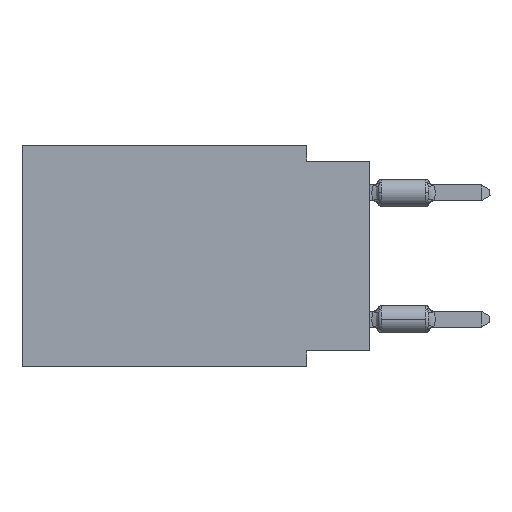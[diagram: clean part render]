
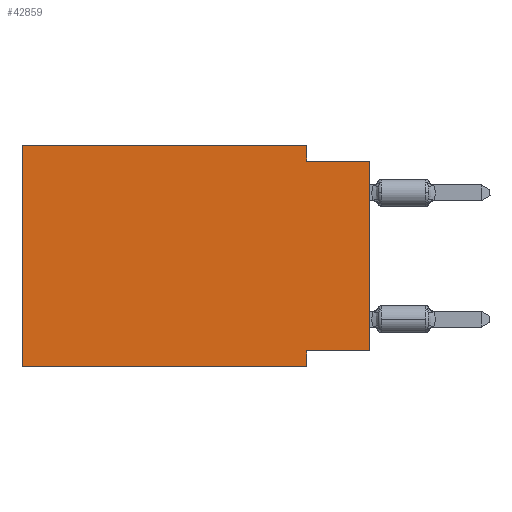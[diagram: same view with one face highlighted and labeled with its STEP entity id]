
A CAD part, left-side view. The second image highlights one B-rep face of the part: STEP entity #42859.
In plain terms, the highlighted planar face has unit normal (-1, 0, 0).
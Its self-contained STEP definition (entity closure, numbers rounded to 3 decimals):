
#439 = VERTEX_POINT ( 'NONE', #24059 ) ;
#2502 = EDGE_CURVE ( 'NONE', #50353, #28682, #31240, .T. ) ;
#2785 = CARTESIAN_POINT ( 'NONE',  ( 0., 0., 0. ) ) ;
#2796 = CARTESIAN_POINT ( 'NONE',  ( 0., 13.97, 0. ) ) ;
#3063 = AXIS2_PLACEMENT_3D ( 'NONE', #2796, #46079, #18125 ) ;
#3185 = CARTESIAN_POINT ( 'NONE',  ( 0., 0., -8.255 ) ) ;
#4720 = EDGE_CURVE ( 'NONE', #48730, #28686, #17129, .T. ) ;
#4770 = CARTESIAN_POINT ( 'NONE',  ( 0., 2.54, -0.635 ) ) ;
#7696 = EDGE_CURVE ( 'NONE', #50228, #50353, #31667, .T. ) ;
#11003 = LINE ( 'NONE', #39218, #25266 ) ;
#14453 = CARTESIAN_POINT ( 'NONE',  ( 0., 13.97, 0. ) ) ;
#14509 = VECTOR ( 'NONE', #24447, 1000. ) ;
#15107 = LINE ( 'NONE', #31175, #27765 ) ;
#17129 = LINE ( 'NONE', #45602, #43668 ) ;
#18125 = DIRECTION ( 'NONE',  ( 0., 0., -1. ) ) ;
#22542 = ORIENTED_EDGE ( 'NONE', *, *, #4720, .F. ) ;
#24059 = CARTESIAN_POINT ( 'NONE',  ( 0., 0., -0.635 ) ) ;
#24447 = DIRECTION ( 'NONE',  ( 0., -1., 0. ) ) ;
#24557 = ORIENTED_EDGE ( 'NONE', *, *, #34786, .F. ) ;
#25266 = VECTOR ( 'NONE', #31302, 1000. ) ;
#25307 = CARTESIAN_POINT ( 'NONE',  ( 0., 13.97, -8.89 ) ) ;
#27765 = VECTOR ( 'NONE', #47256, 1000. ) ;
#28682 = VERTEX_POINT ( 'NONE', #49790 ) ;
#28686 = VERTEX_POINT ( 'NONE', #14453 ) ;
#29984 = FACE_OUTER_BOUND ( 'NONE', #46580, .T. ) ;
#30478 = DIRECTION ( 'NONE',  ( 0., 0., 1. ) ) ;
#31080 = EDGE_CURVE ( 'NONE', #48730, #28682, #40788, .T. ) ;
#31090 = ORIENTED_EDGE ( 'NONE', *, *, #33074, .F. ) ;
#31175 = CARTESIAN_POINT ( 'NONE',  ( 0., 2.54, 0. ) ) ;
#31240 = LINE ( 'NONE', #50745, #32575 ) ;
#31302 = DIRECTION ( 'NONE',  ( 0., -1., 0. ) ) ;
#31667 = LINE ( 'NONE', #3185, #40478 ) ;
#32575 = VECTOR ( 'NONE', #46552, 1000. ) ;
#33074 = EDGE_CURVE ( 'NONE', #28686, #51881, #40324, .T. ) ;
#33161 = VECTOR ( 'NONE', #47181, 1000. ) ;
#33210 = DIRECTION ( 'NONE',  ( 0., 0., 1. ) ) ;
#34425 = EDGE_CURVE ( 'NONE', #51881, #49497, #15107, .T. ) ;
#34786 = EDGE_CURVE ( 'NONE', #49497, #439, #11003, .T. ) ;
#38143 = LINE ( 'NONE', #2785, #42361 ) ;
#38491 = ORIENTED_EDGE ( 'NONE', *, *, #7696, .F. ) ;
#39218 = CARTESIAN_POINT ( 'NONE',  ( 0., 0., -0.635 ) ) ;
#39727 = CARTESIAN_POINT ( 'NONE',  ( 0., 2.54, -8.255 ) ) ;
#40324 = LINE ( 'NONE', #51388, #33161 ) ;
#40423 = EDGE_CURVE ( 'NONE', #50228, #439, #38143, .T. ) ;
#40478 = VECTOR ( 'NONE', #42759, 1000. ) ;
#40562 = ORIENTED_EDGE ( 'NONE', *, *, #34425, .F. ) ;
#40788 = LINE ( 'NONE', #44490, #14509 ) ;
#42361 = VECTOR ( 'NONE', #30478, 1000. ) ;
#42759 = DIRECTION ( 'NONE',  ( 0., 1., 0. ) ) ;
#42859 = ADVANCED_FACE ( 'NONE', ( #29984 ), #51046, .F. ) ;
#43668 = VECTOR ( 'NONE', #33210, 1000. ) ;
#44490 = CARTESIAN_POINT ( 'NONE',  ( 0., 13.97, -8.89 ) ) ;
#45602 = CARTESIAN_POINT ( 'NONE',  ( 0., 13.97, 0. ) ) ;
#46079 = DIRECTION ( 'NONE',  ( 1., 0., 0. ) ) ;
#46296 = CARTESIAN_POINT ( 'NONE',  ( 0., 2.54, 0. ) ) ;
#46552 = DIRECTION ( 'NONE',  ( 0., 0., -1. ) ) ;
#46580 = EDGE_LOOP ( 'NONE', ( #52095, #24557, #40562, #31090, #22542, #47727, #51848, #38491 ) ) ;
#47181 = DIRECTION ( 'NONE',  ( 0., -1., 0. ) ) ;
#47256 = DIRECTION ( 'NONE',  ( 0., 0., -1. ) ) ;
#47370 = CARTESIAN_POINT ( 'NONE',  ( 0., 0., -8.255 ) ) ;
#47727 = ORIENTED_EDGE ( 'NONE', *, *, #31080, .T. ) ;
#48730 = VERTEX_POINT ( 'NONE', #25307 ) ;
#49497 = VERTEX_POINT ( 'NONE', #4770 ) ;
#49790 = CARTESIAN_POINT ( 'NONE',  ( 0., 2.54, -8.89 ) ) ;
#50228 = VERTEX_POINT ( 'NONE', #47370 ) ;
#50353 = VERTEX_POINT ( 'NONE', #39727 ) ;
#50745 = CARTESIAN_POINT ( 'NONE',  ( 0., 2.54, -8.89 ) ) ;
#51046 = PLANE ( 'NONE',  #3063 ) ;
#51388 = CARTESIAN_POINT ( 'NONE',  ( 0., 13.97, 0. ) ) ;
#51848 = ORIENTED_EDGE ( 'NONE', *, *, #2502, .F. ) ;
#51881 = VERTEX_POINT ( 'NONE', #46296 ) ;
#52095 = ORIENTED_EDGE ( 'NONE', *, *, #40423, .T. ) ;
